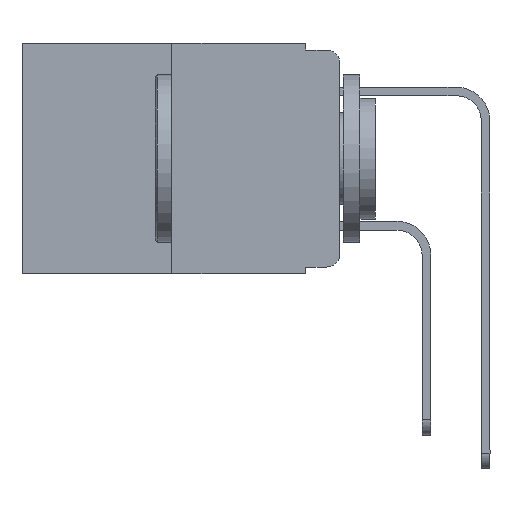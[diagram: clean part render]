
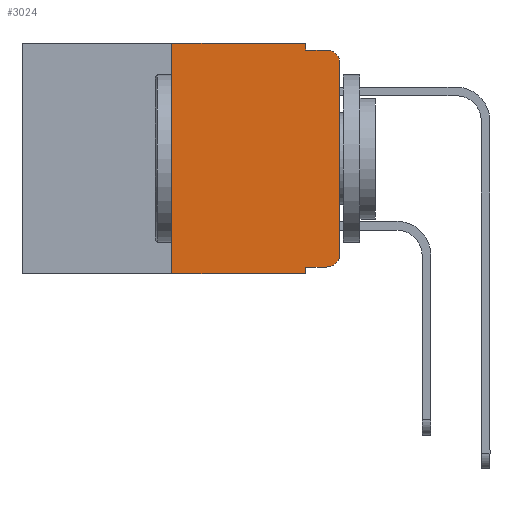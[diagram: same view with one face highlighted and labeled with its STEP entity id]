
A CAD part, left-side view. The second image highlights one B-rep face of the part: STEP entity #3024.
In plain terms, the highlighted planar face has unit normal (-1, 0, 0).
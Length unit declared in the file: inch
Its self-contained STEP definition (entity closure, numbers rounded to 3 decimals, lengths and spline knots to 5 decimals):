
#28 = CARTESIAN_POINT ( 'NONE',  ( 0., 0., -0.03 ) ) ;
#76 = DIRECTION ( 'NONE',  ( 0., 0., 1. ) ) ;
#77 = CARTESIAN_POINT ( 'NONE',  ( 0., 0.25, 0. ) ) ;
#125 = CARTESIAN_POINT ( 'NONE',  ( 0., 0.473, 0. ) ) ;
#305 = EDGE_LOOP ( 'NONE', ( #2866, #15838, #7929, #12694, #20700, #10166, #19033, #18445, #10047, #8321 ) ) ;
#363 = DIRECTION ( 'NONE',  ( 1., 0., 0. ) ) ;
#470 = DIRECTION ( 'NONE',  ( 0., -1., 0. ) ) ;
#471 = CIRCLE ( 'NONE', #20254, 0.02 ) ;
#499 = EDGE_CURVE ( 'NONE', #13829, #3531, #10191, .T. ) ;
#1847 = DIRECTION ( 'NONE',  ( 0., 0., -1. ) ) ;
#2317 = CARTESIAN_POINT ( 'NONE',  ( 0., 0.051, 0. ) ) ;
#2536 = LINE ( 'NONE', #15327, #4055 ) ;
#2580 = CARTESIAN_POINT ( 'NONE',  ( 0., 0.02, -0.333 ) ) ;
#2618 = LINE ( 'NONE', #18767, #6882 ) ;
#2823 = DIRECTION ( 'NONE',  ( 0., -1., 0. ) ) ;
#2866 = ORIENTED_EDGE ( 'NONE', *, *, #2907, .T. ) ;
#2907 = EDGE_CURVE ( 'NONE', #3531, #5444, #10788, .T. ) ;
#3024 = ADVANCED_FACE ( 'NONE', ( #11513 ), #4896, .F. ) ;
#3453 = EDGE_CURVE ( 'NONE', #11190, #17206, #4965, .T. ) ;
#3531 = VERTEX_POINT ( 'NONE', #3865 ) ;
#3730 = CARTESIAN_POINT ( 'NONE',  ( 0., 0.473, 0. ) ) ;
#3865 = CARTESIAN_POINT ( 'NONE',  ( 0., 0., -0.313 ) ) ;
#4055 = VECTOR ( 'NONE', #17501, 39.37008 ) ;
#4170 = LINE ( 'NONE', #16851, #6176 ) ;
#4896 = PLANE ( 'NONE',  #13566 ) ;
#4965 = LINE ( 'NONE', #125, #18015 ) ;
#5444 = VERTEX_POINT ( 'NONE', #28 ) ;
#6176 = VECTOR ( 'NONE', #470, 39.37008 ) ;
#6566 = CARTESIAN_POINT ( 'NONE',  ( 0., 0.02, -0.313 ) ) ;
#6579 = DIRECTION ( 'NONE',  ( -1., 0., 0. ) ) ;
#6882 = VECTOR ( 'NONE', #2823, 39.37008 ) ;
#7142 = DIRECTION ( 'NONE',  ( 0., 0., -1. ) ) ;
#7929 = ORIENTED_EDGE ( 'NONE', *, *, #20613, .F. ) ;
#7938 = CARTESIAN_POINT ( 'NONE',  ( 0., 0.02, -0.03 ) ) ;
#8046 = EDGE_CURVE ( 'NONE', #11001, #10683, #2536, .T. ) ;
#8105 = LINE ( 'NONE', #17753, #18145 ) ;
#8177 = AXIS2_PLACEMENT_3D ( 'NONE', #6566, #11306, #17682 ) ;
#8237 = DIRECTION ( 'NONE',  ( 0., -1., 0. ) ) ;
#8321 = ORIENTED_EDGE ( 'NONE', *, *, #499, .T. ) ;
#8474 = LINE ( 'NONE', #14769, #12566 ) ;
#8500 = VECTOR ( 'NONE', #11101, 39.37008 ) ;
#8589 = CARTESIAN_POINT ( 'NONE',  ( 0., 0.051, -0.01 ) ) ;
#9127 = EDGE_CURVE ( 'NONE', #17206, #20228, #8105, .T. ) ;
#9419 = CARTESIAN_POINT ( 'NONE',  ( 0., 0., 0. ) ) ;
#9604 = VERTEX_POINT ( 'NONE', #19508 ) ;
#9813 = LINE ( 'NONE', #17878, #17264 ) ;
#10047 = ORIENTED_EDGE ( 'NONE', *, *, #17701, .T. ) ;
#10166 = ORIENTED_EDGE ( 'NONE', *, *, #13002, .F. ) ;
#10191 = CIRCLE ( 'NONE', #8177, 0.02 ) ;
#10683 = VERTEX_POINT ( 'NONE', #14080 ) ;
#10788 = LINE ( 'NONE', #9419, #8500 ) ;
#11001 = VERTEX_POINT ( 'NONE', #16888 ) ;
#11064 = VERTEX_POINT ( 'NONE', #20349 ) ;
#11101 = DIRECTION ( 'NONE',  ( 0., 0., 1. ) ) ;
#11190 = VERTEX_POINT ( 'NONE', #77 ) ;
#11306 = DIRECTION ( 'NONE',  ( -1., 0., 0. ) ) ;
#11513 = FACE_OUTER_BOUND ( 'NONE', #305, .T. ) ;
#12566 = VECTOR ( 'NONE', #76, 39.37008 ) ;
#12694 = ORIENTED_EDGE ( 'NONE', *, *, #9127, .F. ) ;
#13002 = EDGE_CURVE ( 'NONE', #11064, #11190, #8474, .T. ) ;
#13431 = EDGE_CURVE ( 'NONE', #5444, #9604, #471, .T. ) ;
#13566 = AXIS2_PLACEMENT_3D ( 'NONE', #3730, #363, #1847 ) ;
#13829 = VERTEX_POINT ( 'NONE', #2580 ) ;
#14080 = CARTESIAN_POINT ( 'NONE',  ( 0., 0.051, -0.343 ) ) ;
#14769 = CARTESIAN_POINT ( 'NONE',  ( 0., 0.25, 0. ) ) ;
#15327 = CARTESIAN_POINT ( 'NONE',  ( 0., 0.051, 0. ) ) ;
#15838 = ORIENTED_EDGE ( 'NONE', *, *, #13431, .T. ) ;
#16083 = DIRECTION ( 'NONE',  ( 0., -1., 0. ) ) ;
#16851 = CARTESIAN_POINT ( 'NONE',  ( 0., 0.051, -0.333 ) ) ;
#16888 = CARTESIAN_POINT ( 'NONE',  ( 0., 0.051, -0.333 ) ) ;
#17206 = VERTEX_POINT ( 'NONE', #2317 ) ;
#17264 = VECTOR ( 'NONE', #8237, 39.37008 ) ;
#17501 = DIRECTION ( 'NONE',  ( 0., 0., -1. ) ) ;
#17682 = DIRECTION ( 'NONE',  ( 0., 0., -1. ) ) ;
#17701 = EDGE_CURVE ( 'NONE', #11001, #13829, #4170, .T. ) ;
#17753 = CARTESIAN_POINT ( 'NONE',  ( 0., 0.051, 0. ) ) ;
#17878 = CARTESIAN_POINT ( 'NONE',  ( 0., 0.051, -0.01 ) ) ;
#18015 = VECTOR ( 'NONE', #16083, 39.37008 ) ;
#18145 = VECTOR ( 'NONE', #7142, 39.37008 ) ;
#18445 = ORIENTED_EDGE ( 'NONE', *, *, #8046, .F. ) ;
#18767 = CARTESIAN_POINT ( 'NONE',  ( 0., 0.473, -0.343 ) ) ;
#19033 = ORIENTED_EDGE ( 'NONE', *, *, #19151, .T. ) ;
#19151 = EDGE_CURVE ( 'NONE', #11064, #10683, #2618, .T. ) ;
#19156 = DIRECTION ( 'NONE',  ( 0., 0., -1. ) ) ;
#19508 = CARTESIAN_POINT ( 'NONE',  ( 0., 0.02, -0.01 ) ) ;
#20228 = VERTEX_POINT ( 'NONE', #8589 ) ;
#20254 = AXIS2_PLACEMENT_3D ( 'NONE', #7938, #6579, #19156 ) ;
#20349 = CARTESIAN_POINT ( 'NONE',  ( 0., 0.25, -0.343 ) ) ;
#20613 = EDGE_CURVE ( 'NONE', #20228, #9604, #9813, .T. ) ;
#20700 = ORIENTED_EDGE ( 'NONE', *, *, #3453, .F. ) ;
